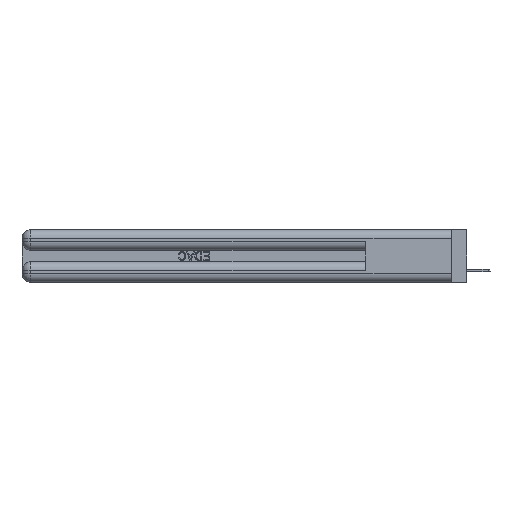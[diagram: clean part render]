
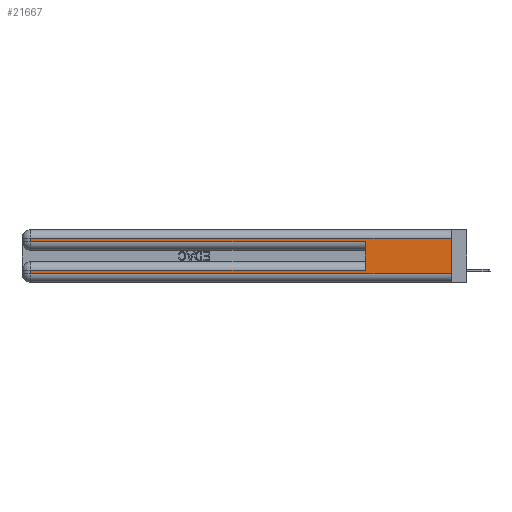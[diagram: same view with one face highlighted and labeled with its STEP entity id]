
A CAD part, left-side view. The second image highlights one B-rep face of the part: STEP entity #21667.
In plain terms, the highlighted planar face has unit normal (-1, 0, 0).
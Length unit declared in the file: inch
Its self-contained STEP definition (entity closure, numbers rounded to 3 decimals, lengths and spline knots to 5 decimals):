
#1164 = VECTOR ( 'NONE', #32639, 39.37008 ) ;
#1483 = EDGE_CURVE ( 'NONE', #23721, #24737, #38015, .T. ) ;
#2412 = CARTESIAN_POINT ( 'NONE',  ( 0., 2.94, 0.06 ) ) ;
#2422 = CARTESIAN_POINT ( 'NONE',  ( 0., 0.6, 0.145 ) ) ;
#2598 = LINE ( 'NONE', #38436, #28775 ) ;
#4457 = EDGE_CURVE ( 'NONE', #16269, #18490, #36781, .T. ) ;
#5131 = EDGE_CURVE ( 'NONE', #13858, #24737, #13341, .T. ) ;
#7319 = LINE ( 'NONE', #29249, #38697 ) ;
#9204 = CARTESIAN_POINT ( 'NONE',  ( 0., 0., 0.085 ) ) ;
#9932 = DIRECTION ( 'NONE',  ( 0., 0., -1. ) ) ;
#10340 = ORIENTED_EDGE ( 'NONE', *, *, #27790, .F. ) ;
#11498 = VERTEX_POINT ( 'NONE', #15351 ) ;
#12225 = CARTESIAN_POINT ( 'NONE',  ( 0., 2.94, 0.085 ) ) ;
#12388 = VECTOR ( 'NONE', #25133, 39.37008 ) ;
#12596 = EDGE_CURVE ( 'NONE', #29813, #13858, #31834, .T. ) ;
#13164 = ORIENTED_EDGE ( 'NONE', *, *, #29536, .T. ) ;
#13341 = LINE ( 'NONE', #19001, #12388 ) ;
#13858 = VERTEX_POINT ( 'NONE', #2412 ) ;
#14366 = DIRECTION ( 'NONE',  ( 0., 1., 0. ) ) ;
#14981 = ORIENTED_EDGE ( 'NONE', *, *, #12596, .T. ) ;
#15351 = CARTESIAN_POINT ( 'NONE',  ( 0., 0.6, 0.085 ) ) ;
#15353 = EDGE_CURVE ( 'NONE', #11498, #29813, #38730, .T. ) ;
#15374 = PLANE ( 'NONE',  #38464 ) ;
#15717 = CARTESIAN_POINT ( 'NONE',  ( 0., 2.94, 0.285 ) ) ;
#16269 = VERTEX_POINT ( 'NONE', #15717 ) ;
#17829 = CARTESIAN_POINT ( 'NONE',  ( 0., 0.6, 0.285 ) ) ;
#18397 = DIRECTION ( 'NONE',  ( 1., 0., 0. ) ) ;
#18490 = VERTEX_POINT ( 'NONE', #17829 ) ;
#19001 = CARTESIAN_POINT ( 'NONE',  ( 0., 0., 0.06 ) ) ;
#20251 = DIRECTION ( 'NONE',  ( 0., 0., -1. ) ) ;
#20375 = EDGE_LOOP ( 'NONE', ( #23376, #13164, #34417, #29102, #10340, #21070, #14981, #38742 ) ) ;
#20421 = CARTESIAN_POINT ( 'NONE',  ( 0., 0., 0.37 ) ) ;
#21070 = ORIENTED_EDGE ( 'NONE', *, *, #15353, .T. ) ;
#21412 = VECTOR ( 'NONE', #32156, 39.37008 ) ;
#21667 = ADVANCED_FACE ( 'NONE', ( #25201 ), #15374, .F. ) ;
#21927 = CARTESIAN_POINT ( 'NONE',  ( 0., 0., 0.285 ) ) ;
#23376 = ORIENTED_EDGE ( 'NONE', *, *, #1483, .F. ) ;
#23721 = VERTEX_POINT ( 'NONE', #37583 ) ;
#24737 = VERTEX_POINT ( 'NONE', #24769 ) ;
#24769 = CARTESIAN_POINT ( 'NONE',  ( 0., 0., 0.06 ) ) ;
#24782 = VECTOR ( 'NONE', #36112, 39.37008 ) ;
#25133 = DIRECTION ( 'NONE',  ( 0., -1., 0. ) ) ;
#25201 = FACE_OUTER_BOUND ( 'NONE', #20375, .T. ) ;
#26031 = VECTOR ( 'NONE', #33584, 39.37008 ) ;
#27790 = EDGE_CURVE ( 'NONE', #11498, #18490, #36878, .T. ) ;
#28703 = VERTEX_POINT ( 'NONE', #34523 ) ;
#28775 = VECTOR ( 'NONE', #20251, 39.37008 ) ;
#29102 = ORIENTED_EDGE ( 'NONE', *, *, #4457, .T. ) ;
#29249 = CARTESIAN_POINT ( 'NONE',  ( 0., 0., 0.31 ) ) ;
#29536 = EDGE_CURVE ( 'NONE', #23721, #28703, #7319, .T. ) ;
#29783 = DIRECTION ( 'NONE',  ( 0., 0., -1. ) ) ;
#29813 = VERTEX_POINT ( 'NONE', #12225 ) ;
#30029 = VECTOR ( 'NONE', #9932, 39.37008 ) ;
#31834 = LINE ( 'NONE', #32849, #24782 ) ;
#32156 = DIRECTION ( 'NONE',  ( 0., 0., 1. ) ) ;
#32639 = DIRECTION ( 'NONE',  ( 0., 1., 0. ) ) ;
#32849 = CARTESIAN_POINT ( 'NONE',  ( 0., 2.94, 0.37 ) ) ;
#33584 = DIRECTION ( 'NONE',  ( 0., -1., 0. ) ) ;
#34417 = ORIENTED_EDGE ( 'NONE', *, *, #35139, .T. ) ;
#34523 = CARTESIAN_POINT ( 'NONE',  ( 0., 2.94, 0.31 ) ) ;
#35139 = EDGE_CURVE ( 'NONE', #28703, #16269, #2598, .T. ) ;
#36112 = DIRECTION ( 'NONE',  ( 0., 0., -1. ) ) ;
#36302 = CARTESIAN_POINT ( 'NONE',  ( 0., 0., 0.37 ) ) ;
#36781 = LINE ( 'NONE', #21927, #26031 ) ;
#36878 = LINE ( 'NONE', #2422, #21412 ) ;
#37583 = CARTESIAN_POINT ( 'NONE',  ( 0., 0., 0.31 ) ) ;
#38015 = LINE ( 'NONE', #20421, #30029 ) ;
#38436 = CARTESIAN_POINT ( 'NONE',  ( 0., 2.94, 0.37 ) ) ;
#38464 = AXIS2_PLACEMENT_3D ( 'NONE', #36302, #18397, #29783 ) ;
#38697 = VECTOR ( 'NONE', #14366, 39.37008 ) ;
#38730 = LINE ( 'NONE', #9204, #1164 ) ;
#38742 = ORIENTED_EDGE ( 'NONE', *, *, #5131, .T. ) ;
